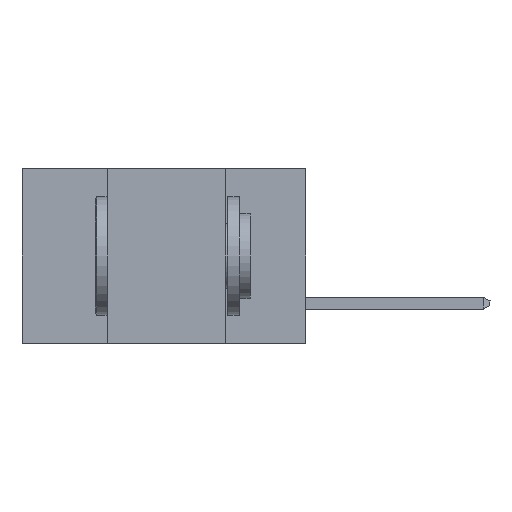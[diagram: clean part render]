
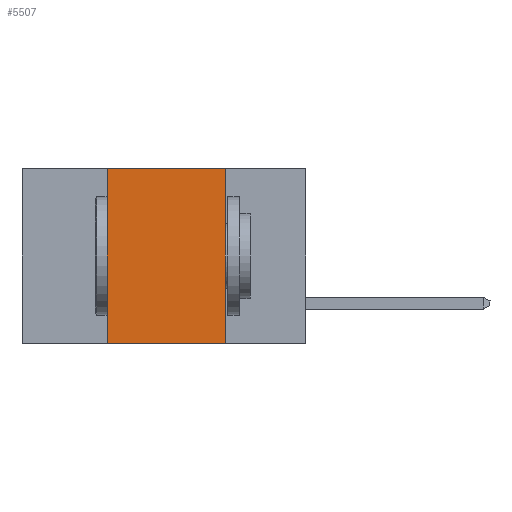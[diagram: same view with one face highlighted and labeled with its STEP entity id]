
A CAD part, left-side view. The second image highlights one B-rep face of the part: STEP entity #5507.
In plain terms, the highlighted planar face has unit normal (-1, 0, 0).
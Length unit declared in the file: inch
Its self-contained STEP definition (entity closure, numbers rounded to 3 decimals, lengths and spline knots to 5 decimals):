
#182 = LINE ( 'NONE', #11399, #12146 ) ;
#1059 = VECTOR ( 'NONE', #6661, 39.37008 ) ;
#1124 = ORIENTED_EDGE ( 'NONE', *, *, #10142, .F. ) ;
#1565 = VERTEX_POINT ( 'NONE', #11734 ) ;
#1770 = ORIENTED_EDGE ( 'NONE', *, *, #14491, .T. ) ;
#2325 = DIRECTION ( 'NONE',  ( 0., 0., -1. ) ) ;
#2562 = CARTESIAN_POINT ( 'NONE',  ( 0., 0.17, -0.37 ) ) ;
#2871 = CARTESIAN_POINT ( 'NONE',  ( 0., 0.42, 0. ) ) ;
#2904 = EDGE_CURVE ( 'NONE', #1565, #4494, #182, .T. ) ;
#3357 = DIRECTION ( 'NONE',  ( 1., 0., 0. ) ) ;
#3395 = ORIENTED_EDGE ( 'NONE', *, *, #9669, .F. ) ;
#4494 = VERTEX_POINT ( 'NONE', #2871 ) ;
#4516 = CARTESIAN_POINT ( 'NONE',  ( 0., 0.6, 0. ) ) ;
#5507 = ADVANCED_FACE ( 'NONE', ( #14823 ), #10217, .F. ) ;
#6661 = DIRECTION ( 'NONE',  ( 0., -1., 0. ) ) ;
#6775 = EDGE_LOOP ( 'NONE', ( #3395, #1124, #9860, #1770 ) ) ;
#7739 = CARTESIAN_POINT ( 'NONE',  ( 0., 0.6, 0. ) ) ;
#7862 = DIRECTION ( 'NONE',  ( 0., 0., -1. ) ) ;
#7914 = VECTOR ( 'NONE', #7862, 39.37008 ) ;
#7981 = DIRECTION ( 'NONE',  ( 0., 0., 1. ) ) ;
#9186 = CARTESIAN_POINT ( 'NONE',  ( 0., 0.17, 0. ) ) ;
#9669 = EDGE_CURVE ( 'NONE', #12219, #12338, #10036, .T. ) ;
#9860 = ORIENTED_EDGE ( 'NONE', *, *, #2904, .F. ) ;
#10036 = LINE ( 'NONE', #14585, #7914 ) ;
#10142 = EDGE_CURVE ( 'NONE', #4494, #12219, #13756, .T. ) ;
#10217 = PLANE ( 'NONE',  #10882 ) ;
#10882 = AXIS2_PLACEMENT_3D ( 'NONE', #4516, #3357, #2325 ) ;
#11399 = CARTESIAN_POINT ( 'NONE',  ( 0., 0.42, 0. ) ) ;
#11558 = LINE ( 'NONE', #14245, #14092 ) ;
#11734 = CARTESIAN_POINT ( 'NONE',  ( 0., 0.42, -0.37 ) ) ;
#12146 = VECTOR ( 'NONE', #7981, 39.37008 ) ;
#12219 = VERTEX_POINT ( 'NONE', #9186 ) ;
#12338 = VERTEX_POINT ( 'NONE', #2562 ) ;
#13756 = LINE ( 'NONE', #7739, #1059 ) ;
#14092 = VECTOR ( 'NONE', #14197, 39.37008 ) ;
#14197 = DIRECTION ( 'NONE',  ( 0., -1., 0. ) ) ;
#14245 = CARTESIAN_POINT ( 'NONE',  ( 0., 0.6, -0.37 ) ) ;
#14491 = EDGE_CURVE ( 'NONE', #1565, #12338, #11558, .T. ) ;
#14585 = CARTESIAN_POINT ( 'NONE',  ( 0., 0.17, 0. ) ) ;
#14823 = FACE_OUTER_BOUND ( 'NONE', #6775, .T. ) ;
